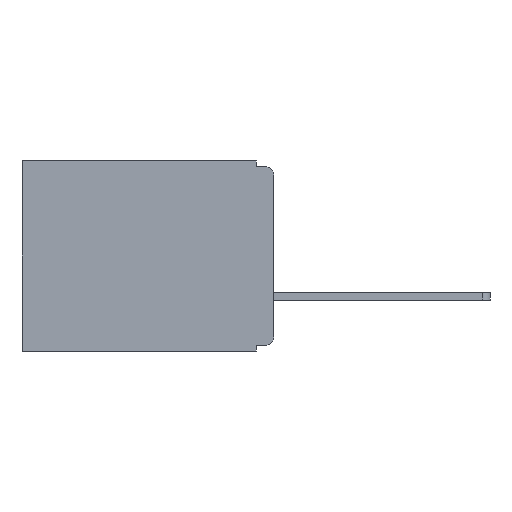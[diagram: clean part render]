
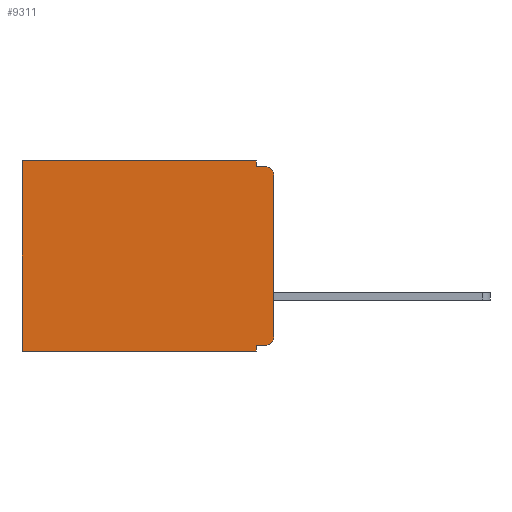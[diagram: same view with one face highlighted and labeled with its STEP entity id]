
A CAD part, left-side view. The second image highlights one B-rep face of the part: STEP entity #9311.
In plain terms, the highlighted planar face has unit normal (-1, 0, 0).
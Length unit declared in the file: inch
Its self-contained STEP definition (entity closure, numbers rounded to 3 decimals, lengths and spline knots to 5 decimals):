
#372 = CARTESIAN_POINT ( 'NONE',  ( 0.3, 0., -0.33 ) ) ;
#1101 = VECTOR ( 'NONE', #7303, 39.37008 ) ;
#1282 = LINE ( 'NONE', #7462, #1101 ) ;
#1298 = VERTEX_POINT ( 'NONE', #11836 ) ;
#1655 = VERTEX_POINT ( 'NONE', #10403 ) ;
#2113 = EDGE_CURVE ( 'NONE', #15938, #8342, #5275, .T. ) ;
#2156 = FACE_OUTER_BOUND ( 'NONE', #6670, .T. ) ;
#2873 = DIRECTION ( 'NONE',  ( 0., 0., -1. ) ) ;
#3499 = VECTOR ( 'NONE', #14496, 39.37008 ) ;
#3612 = LINE ( 'NONE', #14203, #3499 ) ;
#4009 = VERTEX_POINT ( 'NONE', #10146 ) ;
#4139 = CARTESIAN_POINT ( 'NONE',  ( 0.3, 0., -0.025 ) ) ;
#5224 = VECTOR ( 'NONE', #10801, 39.37008 ) ;
#5275 = LINE ( 'NONE', #10411, #5224 ) ;
#5523 = VECTOR ( 'NONE', #2873, 39.37008 ) ;
#5552 = LINE ( 'NONE', #7909, #5523 ) ;
#5642 = CARTESIAN_POINT ( 'NONE',  ( 0.3, 0.031, -0.33 ) ) ;
#6118 = VERTEX_POINT ( 'NONE', #6740 ) ;
#6207 = CARTESIAN_POINT ( 'NONE',  ( 0.3, 0.031, 0. ) ) ;
#6614 = DIRECTION ( 'NONE',  ( 0., 0., -1. ) ) ;
#6670 = EDGE_LOOP ( 'NONE', ( #14014, #14862, #13805, #9969, #11349, #11444, #12497, #15805, #11505, #11671 ) ) ;
#6740 = CARTESIAN_POINT ( 'NONE',  ( 0.3, 0., -0.305 ) ) ;
#6855 = CARTESIAN_POINT ( 'NONE',  ( 0.3, 0.015, -0.32 ) ) ;
#7077 = DIRECTION ( 'NONE',  ( 0., 0., -1. ) ) ;
#7202 = DIRECTION ( 'NONE',  ( -1., 0., 0. ) ) ;
#7303 = DIRECTION ( 'NONE',  ( 0., 1., 0. ) ) ;
#7442 = CARTESIAN_POINT ( 'NONE',  ( 0.3, 0.437, 0. ) ) ;
#7462 = CARTESIAN_POINT ( 'NONE',  ( 0.3, 0., -0.32 ) ) ;
#7605 = CARTESIAN_POINT ( 'NONE',  ( 0.3, 0.015, -0.025 ) ) ;
#7904 = AXIS2_PLACEMENT_3D ( 'NONE', #13073, #13059, #13043 ) ;
#7909 = CARTESIAN_POINT ( 'NONE',  ( 0.3, 0., -0.33 ) ) ;
#8342 = VERTEX_POINT ( 'NONE', #7442 ) ;
#8445 = EDGE_CURVE ( 'NONE', #13812, #6118, #5552, .T. ) ;
#8980 = EDGE_CURVE ( 'NONE', #4009, #11604, #3612, .T. ) ;
#9311 = ADVANCED_FACE ( 'NONE', ( #2156 ), #13280, .F. ) ;
#9339 = VERTEX_POINT ( 'NONE', #12050 ) ;
#9579 = EDGE_CURVE ( 'NONE', #13196, #1655, #1282, .T. ) ;
#9674 = AXIS2_PLACEMENT_3D ( 'NONE', #7605, #7202, #7077 ) ;
#9888 = EDGE_CURVE ( 'NONE', #1298, #9339, #13888, .T. ) ;
#9969 = ORIENTED_EDGE ( 'NONE', *, *, #14110, .F. ) ;
#10022 = EDGE_CURVE ( 'NONE', #13812, #11604, #12989, .T. ) ;
#10088 = VECTOR ( 'NONE', #16572, 39.37008 ) ;
#10146 = CARTESIAN_POINT ( 'NONE',  ( 0.3, 0.031, -0.01 ) ) ;
#10240 = EDGE_CURVE ( 'NONE', #13196, #6118, #11021, .T. ) ;
#10403 = CARTESIAN_POINT ( 'NONE',  ( 0.3, 0.031, -0.32 ) ) ;
#10411 = CARTESIAN_POINT ( 'NONE',  ( 0.3, 0., 0. ) ) ;
#10707 = DIRECTION ( 'NONE',  ( 0., 0., -1. ) ) ;
#10788 = CARTESIAN_POINT ( 'NONE',  ( 0.3, 0.437, -0.33 ) ) ;
#10801 = DIRECTION ( 'NONE',  ( 0., 1., 0. ) ) ;
#11021 = CIRCLE ( 'NONE', #7904, 0.015 ) ;
#11349 = ORIENTED_EDGE ( 'NONE', *, *, #2113, .T. ) ;
#11444 = ORIENTED_EDGE ( 'NONE', *, *, #16611, .T. ) ;
#11505 = ORIENTED_EDGE ( 'NONE', *, *, #9579, .F. ) ;
#11604 = VERTEX_POINT ( 'NONE', #15967 ) ;
#11671 = ORIENTED_EDGE ( 'NONE', *, *, #10240, .T. ) ;
#11836 = CARTESIAN_POINT ( 'NONE',  ( 0.3, 0.031, -0.33 ) ) ;
#11872 = LINE ( 'NONE', #16645, #10088 ) ;
#12050 = CARTESIAN_POINT ( 'NONE',  ( 0.3, 0.437, -0.33 ) ) ;
#12497 = ORIENTED_EDGE ( 'NONE', *, *, #9888, .F. ) ;
#12680 = DIRECTION ( 'NONE',  ( 0., 0., -1. ) ) ;
#12693 = DIRECTION ( 'NONE',  ( 1., 0., 0. ) ) ;
#12708 = CARTESIAN_POINT ( 'NONE',  ( 0.3, 0., -0.33 ) ) ;
#12989 = CIRCLE ( 'NONE', #9674, 0.015 ) ;
#13043 = DIRECTION ( 'NONE',  ( 0., 0., -1. ) ) ;
#13059 = DIRECTION ( 'NONE',  ( -1., 0., 0. ) ) ;
#13073 = CARTESIAN_POINT ( 'NONE',  ( 0.3, 0.015, -0.305 ) ) ;
#13196 = VERTEX_POINT ( 'NONE', #6855 ) ;
#13280 = PLANE ( 'NONE',  #15154 ) ;
#13805 = ORIENTED_EDGE ( 'NONE', *, *, #8980, .F. ) ;
#13812 = VERTEX_POINT ( 'NONE', #4139 ) ;
#13888 = LINE ( 'NONE', #372, #13930 ) ;
#13930 = VECTOR ( 'NONE', #16470, 39.37008 ) ;
#13962 = LINE ( 'NONE', #10788, #14030 ) ;
#14014 = ORIENTED_EDGE ( 'NONE', *, *, #8445, .F. ) ;
#14030 = VECTOR ( 'NONE', #10707, 39.37008 ) ;
#14110 = EDGE_CURVE ( 'NONE', #15938, #4009, #11872, .T. ) ;
#14203 = CARTESIAN_POINT ( 'NONE',  ( 0.3, 0., -0.01 ) ) ;
#14439 = EDGE_CURVE ( 'NONE', #1655, #1298, #16173, .T. ) ;
#14496 = DIRECTION ( 'NONE',  ( 0., -1., 0. ) ) ;
#14862 = ORIENTED_EDGE ( 'NONE', *, *, #10022, .T. ) ;
#14894 = VECTOR ( 'NONE', #6614, 39.37008 ) ;
#15154 = AXIS2_PLACEMENT_3D ( 'NONE', #12708, #12693, #12680 ) ;
#15805 = ORIENTED_EDGE ( 'NONE', *, *, #14439, .F. ) ;
#15938 = VERTEX_POINT ( 'NONE', #6207 ) ;
#15967 = CARTESIAN_POINT ( 'NONE',  ( 0.3, 0.015, -0.01 ) ) ;
#16173 = LINE ( 'NONE', #5642, #14894 ) ;
#16470 = DIRECTION ( 'NONE',  ( 0., 1., 0. ) ) ;
#16572 = DIRECTION ( 'NONE',  ( 0., 0., -1. ) ) ;
#16611 = EDGE_CURVE ( 'NONE', #8342, #9339, #13962, .T. ) ;
#16645 = CARTESIAN_POINT ( 'NONE',  ( 0.3, 0.031, 0. ) ) ;
